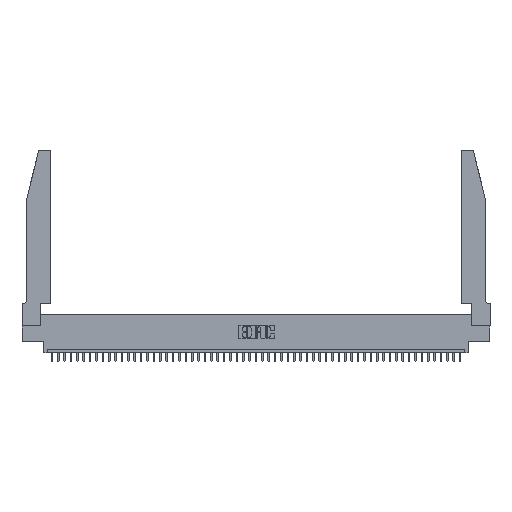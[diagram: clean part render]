
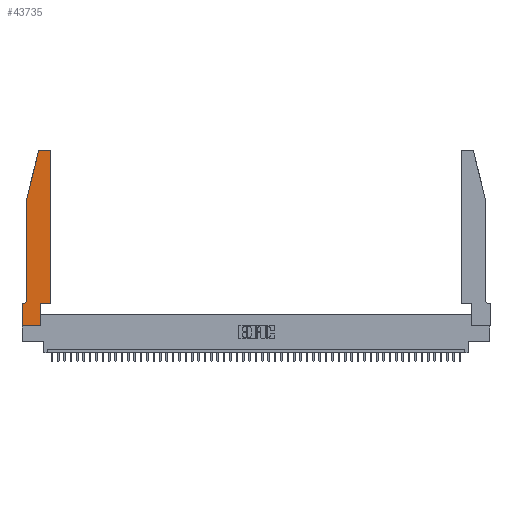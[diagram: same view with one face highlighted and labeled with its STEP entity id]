
A CAD part, top view. The second image highlights one B-rep face of the part: STEP entity #43735.
In plain terms, the highlighted planar face has unit normal (0, 0, 1).
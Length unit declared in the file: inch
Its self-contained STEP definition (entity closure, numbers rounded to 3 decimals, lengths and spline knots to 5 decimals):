
#150 = CARTESIAN_POINT ( 'NONE',  ( 0., 0., 0.37 ) ) ;
#4142 = EDGE_CURVE ( 'NONE', #22794, #41849, #27861, .T. ) ;
#4765 = ORIENTED_EDGE ( 'NONE', *, *, #40987, .T. ) ;
#5185 = CARTESIAN_POINT ( 'NONE',  ( 0.0755, 2., 0.37 ) ) ;
#5312 = CARTESIAN_POINT ( 'NONE',  ( 0.4205, 2.72, 0.37 ) ) ;
#5442 = EDGE_CURVE ( 'NONE', #47211, #21793, #46857, .T. ) ;
#5708 = CIRCLE ( 'NONE', #8660, 0.03 ) ;
#6707 = DIRECTION ( 'NONE',  ( 0., 0., 1. ) ) ;
#7038 = DIRECTION ( 'NONE',  ( 1., 0., 0. ) ) ;
#7044 = EDGE_CURVE ( 'NONE', #15290, #48919, #43001, .T. ) ;
#8275 = ORIENTED_EDGE ( 'NONE', *, *, #4142, .T. ) ;
#8660 = AXIS2_PLACEMENT_3D ( 'NONE', #5312, #21528, #21186 ) ;
#10042 = EDGE_LOOP ( 'NONE', ( #35109, #17368, #39488, #4765, #8275, #42896, #37822, #21715, #24062, #27594, #25238, #50645 ) ) ;
#10148 = CARTESIAN_POINT ( 'NONE',  ( 0.4505, 0.35, 0.37 ) ) ;
#11034 = VERTEX_POINT ( 'NONE', #5185 ) ;
#11631 = DIRECTION ( 'NONE',  ( 0., 0., -1. ) ) ;
#12850 = VERTEX_POINT ( 'NONE', #37979 ) ;
#14821 = AXIS2_PLACEMENT_3D ( 'NONE', #37353, #17300, #29464 ) ;
#15210 = CARTESIAN_POINT ( 'NONE',  ( 0.0055, 0.42, 0.37 ) ) ;
#15290 = VERTEX_POINT ( 'NONE', #21650 ) ;
#15822 = VECTOR ( 'NONE', #23421, 39.37008 ) ;
#16112 = EDGE_CURVE ( 'NONE', #12850, #18185, #30381, .T. ) ;
#16308 = VERTEX_POINT ( 'NONE', #39219 ) ;
#16640 = EDGE_CURVE ( 'NONE', #46066, #12850, #28234, .T. ) ;
#17300 = DIRECTION ( 'NONE',  ( 0., 0., 1. ) ) ;
#17308 = CARTESIAN_POINT ( 'NONE',  ( 0., 0., 0.37 ) ) ;
#17368 = ORIENTED_EDGE ( 'NONE', *, *, #7044, .T. ) ;
#18106 = CARTESIAN_POINT ( 'NONE',  ( 0.2865, 0.35, 0.37 ) ) ;
#18185 = VERTEX_POINT ( 'NONE', #32949 ) ;
#19289 = EDGE_CURVE ( 'NONE', #23624, #47211, #27678, .T. ) ;
#21055 = CARTESIAN_POINT ( 'NONE',  ( 0.2865, 0.35, 0.37 ) ) ;
#21186 = DIRECTION ( 'NONE',  ( 1., 0., 0. ) ) ;
#21336 = VECTOR ( 'NONE', #26304, 39.37008 ) ;
#21528 = DIRECTION ( 'NONE',  ( 0., 0., 1. ) ) ;
#21650 = CARTESIAN_POINT ( 'NONE',  ( 0.284, 2.75, 0.37 ) ) ;
#21715 = ORIENTED_EDGE ( 'NONE', *, *, #5442, .T. ) ;
#21793 = VERTEX_POINT ( 'NONE', #41366 ) ;
#22794 = VERTEX_POINT ( 'NONE', #33153 ) ;
#23421 = DIRECTION ( 'NONE',  ( -0.239, -0.971, 0. ) ) ;
#23624 = VERTEX_POINT ( 'NONE', #50578 ) ;
#23685 = DIRECTION ( 'NONE',  ( -1., 0., 0. ) ) ;
#23717 = AXIS2_PLACEMENT_3D ( 'NONE', #15210, #11631, #42949 ) ;
#24062 = ORIENTED_EDGE ( 'NONE', *, *, #30494, .T. ) ;
#25238 = ORIENTED_EDGE ( 'NONE', *, *, #16112, .T. ) ;
#25449 = VECTOR ( 'NONE', #39402, 39.37008 ) ;
#25685 = DIRECTION ( 'NONE',  ( 0., 1., 0. ) ) ;
#26242 = LINE ( 'NONE', #18106, #21336 ) ;
#26304 = DIRECTION ( 'NONE',  ( 0., 1., 0. ) ) ;
#26318 = CARTESIAN_POINT ( 'NONE',  ( 0.284, 2.72, 0.37 ) ) ;
#27101 = AXIS2_PLACEMENT_3D ( 'NONE', #26318, #6707, #7038 ) ;
#27594 = ORIENTED_EDGE ( 'NONE', *, *, #16640, .T. ) ;
#27678 = LINE ( 'NONE', #150, #43005 ) ;
#27861 = CIRCLE ( 'NONE', #23717, 0.07 ) ;
#28234 = LINE ( 'NONE', #31624, #36193 ) ;
#29464 = DIRECTION ( 'NONE',  ( 1., 0., 0. ) ) ;
#30381 = LINE ( 'NONE', #10148, #34624 ) ;
#30494 = EDGE_CURVE ( 'NONE', #21793, #46066, #26242, .T. ) ;
#31532 = CARTESIAN_POINT ( 'NONE',  ( 0.0055, 0.35, 0.37 ) ) ;
#31624 = CARTESIAN_POINT ( 'NONE',  ( 0.4505, 0.35, 0.37 ) ) ;
#31724 = EDGE_CURVE ( 'NONE', #41849, #23624, #37130, .T. ) ;
#32858 = PLANE ( 'NONE',  #14821 ) ;
#32949 = CARTESIAN_POINT ( 'NONE',  ( 0.4505, 2.72, 0.37 ) ) ;
#33153 = CARTESIAN_POINT ( 'NONE',  ( 0.0755, 0.42, 0.37 ) ) ;
#33184 = VECTOR ( 'NONE', #42282, 39.37008 ) ;
#34347 = CARTESIAN_POINT ( 'NONE',  ( 0.0755, 2., 0.37 ) ) ;
#34624 = VECTOR ( 'NONE', #25685, 39.37008 ) ;
#34988 = LINE ( 'NONE', #34347, #33184 ) ;
#35008 = CARTESIAN_POINT ( 'NONE',  ( 0.2605, 2.75, 0.37 ) ) ;
#35109 = ORIENTED_EDGE ( 'NONE', *, *, #41079, .T. ) ;
#36117 = CARTESIAN_POINT ( 'NONE',  ( 0.0755, 0.35, 0.37 ) ) ;
#36193 = VECTOR ( 'NONE', #48054, 39.37008 ) ;
#37130 = LINE ( 'NONE', #36117, #25449 ) ;
#37353 = CARTESIAN_POINT ( 'NONE',  ( 0., 0.35, 0.37 ) ) ;
#37822 = ORIENTED_EDGE ( 'NONE', *, *, #19289, .T. ) ;
#37979 = CARTESIAN_POINT ( 'NONE',  ( 0.4505, 0.35, 0.37 ) ) ;
#38835 = DIRECTION ( 'NONE',  ( 0., -1., 0. ) ) ;
#39219 = CARTESIAN_POINT ( 'NONE',  ( 0.4205, 2.75, 0.37 ) ) ;
#39402 = DIRECTION ( 'NONE',  ( -1., 0., 0. ) ) ;
#39488 = ORIENTED_EDGE ( 'NONE', *, *, #49349, .T. ) ;
#40431 = CARTESIAN_POINT ( 'NONE',  ( 0.25487, 2.72718, 0.37 ) ) ;
#40519 = VECTOR ( 'NONE', #23685, 39.37008 ) ;
#40987 = EDGE_CURVE ( 'NONE', #11034, #22794, #34988, .T. ) ;
#41079 = EDGE_CURVE ( 'NONE', #16308, #15290, #44839, .T. ) ;
#41366 = CARTESIAN_POINT ( 'NONE',  ( 0.2865, 0., 0.37 ) ) ;
#41849 = VERTEX_POINT ( 'NONE', #31532 ) ;
#42282 = DIRECTION ( 'NONE',  ( 0., -1., 0. ) ) ;
#42673 = FACE_OUTER_BOUND ( 'NONE', #10042, .T. ) ;
#42896 = ORIENTED_EDGE ( 'NONE', *, *, #31724, .T. ) ;
#42949 = DIRECTION ( 'NONE',  ( -1., 0., 0. ) ) ;
#43001 = CIRCLE ( 'NONE', #27101, 0.03 ) ;
#43005 = VECTOR ( 'NONE', #38835, 39.37008 ) ;
#43735 = ADVANCED_FACE ( 'NONE', ( #42673 ), #32858, .T. ) ;
#44397 = VECTOR ( 'NONE', #44724, 39.37008 ) ;
#44432 = CARTESIAN_POINT ( 'NONE',  ( 0., 0., 0.37 ) ) ;
#44724 = DIRECTION ( 'NONE',  ( 1., 0., 0. ) ) ;
#44839 = LINE ( 'NONE', #35008, #40519 ) ;
#46066 = VERTEX_POINT ( 'NONE', #21055 ) ;
#46621 = EDGE_CURVE ( 'NONE', #18185, #16308, #5708, .T. ) ;
#46857 = LINE ( 'NONE', #17308, #44397 ) ;
#46920 = CARTESIAN_POINT ( 'NONE',  ( 0.0755, 2., 0.37 ) ) ;
#47091 = LINE ( 'NONE', #46920, #15822 ) ;
#47211 = VERTEX_POINT ( 'NONE', #44432 ) ;
#48054 = DIRECTION ( 'NONE',  ( 1., 0., 0. ) ) ;
#48919 = VERTEX_POINT ( 'NONE', #40431 ) ;
#49349 = EDGE_CURVE ( 'NONE', #48919, #11034, #47091, .T. ) ;
#50578 = CARTESIAN_POINT ( 'NONE',  ( 0., 0.35, 0.37 ) ) ;
#50645 = ORIENTED_EDGE ( 'NONE', *, *, #46621, .T. ) ;
